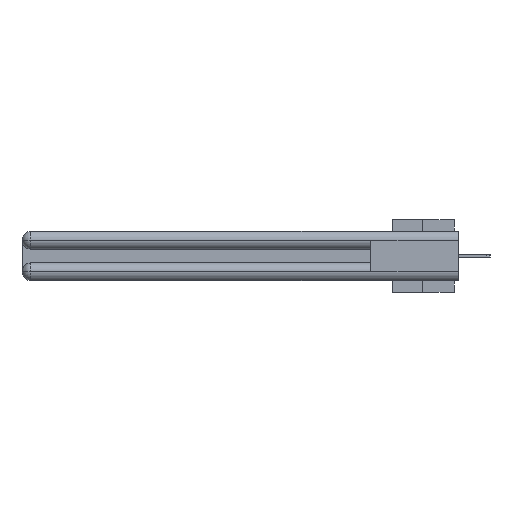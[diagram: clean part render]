
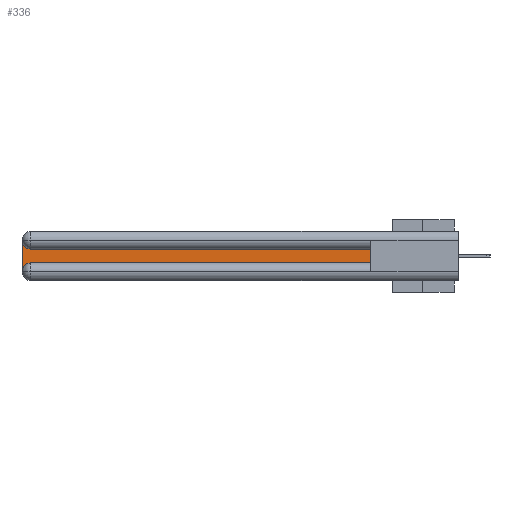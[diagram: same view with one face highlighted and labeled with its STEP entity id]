
A CAD part, left-side view. The second image highlights one B-rep face of the part: STEP entity #336.
In plain terms, the highlighted planar face has unit normal (-1, 0, 0).
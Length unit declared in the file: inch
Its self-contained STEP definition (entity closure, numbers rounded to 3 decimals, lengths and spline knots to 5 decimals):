
#25 = CARTESIAN_POINT ( 'NONE',  ( 0.075, 0.6, -0.1225 ) ) ;
#336 = ADVANCED_FACE ( 'NONE', ( #11092 ), #5457, .F. ) ;
#1108 = DIRECTION ( 'NONE',  ( 1., 0., 0. ) ) ;
#1518 = CARTESIAN_POINT ( 'NONE',  ( 0.075, 3., -0.2175 ) ) ;
#2040 = VERTEX_POINT ( 'NONE', #36958 ) ;
#2284 = DIRECTION ( 'NONE',  ( 1., 0., 0. ) ) ;
#3567 = AXIS2_PLACEMENT_3D ( 'NONE', #16871, #2284, #28264 ) ;
#3638 = VERTEX_POINT ( 'NONE', #27230 ) ;
#3809 = EDGE_CURVE ( 'NONE', #14253, #11996, #15241, .T. ) ;
#4348 = VECTOR ( 'NONE', #9037, 39.37008 ) ;
#4465 = AXIS2_PLACEMENT_3D ( 'NONE', #14529, #25917, #8928 ) ;
#4988 = LINE ( 'NONE', #19565, #5238 ) ;
#5238 = VECTOR ( 'NONE', #22182, 39.37008 ) ;
#5457 = PLANE ( 'NONE',  #3567 ) ;
#5647 = LINE ( 'NONE', #25, #4348 ) ;
#6392 = VECTOR ( 'NONE', #19463, 39.37008 ) ;
#6591 = EDGE_LOOP ( 'NONE', ( #22921, #15003, #34707, #36539, #18831, #24541 ) ) ;
#8928 = DIRECTION ( 'NONE',  ( 0., 0., -1. ) ) ;
#9037 = DIRECTION ( 'NONE',  ( 0., 1., 0. ) ) ;
#9406 = AXIS2_PLACEMENT_3D ( 'NONE', #12530, #1108, #18312 ) ;
#9420 = LINE ( 'NONE', #1518, #22426 ) ;
#10145 = DIRECTION ( 'NONE',  ( 0., 0., -1. ) ) ;
#11092 = FACE_OUTER_BOUND ( 'NONE', #6591, .T. ) ;
#11996 = VERTEX_POINT ( 'NONE', #25471 ) ;
#12530 = CARTESIAN_POINT ( 'NONE',  ( 0.075, 2.94, -0.2775 ) ) ;
#13354 = EDGE_CURVE ( 'NONE', #3638, #21829, #29062, .T. ) ;
#14253 = VERTEX_POINT ( 'NONE', #21542 ) ;
#14529 = CARTESIAN_POINT ( 'NONE',  ( 0.075, 2.94, -0.0625 ) ) ;
#15003 = ORIENTED_EDGE ( 'NONE', *, *, #3809, .T. ) ;
#15241 = CIRCLE ( 'NONE', #4465, 0.06 ) ;
#16393 = EDGE_CURVE ( 'NONE', #34853, #2040, #4988, .T. ) ;
#16871 = CARTESIAN_POINT ( 'NONE',  ( 0.075, 3., -0.1225 ) ) ;
#18312 = DIRECTION ( 'NONE',  ( 0., 0., -1. ) ) ;
#18831 = ORIENTED_EDGE ( 'NONE', *, *, #23660, .T. ) ;
#18912 = CARTESIAN_POINT ( 'NONE',  ( 0.075, 0.6, -0.2175 ) ) ;
#19463 = DIRECTION ( 'NONE',  ( 0., -1., 0. ) ) ;
#19565 = CARTESIAN_POINT ( 'NONE',  ( 0.075, 0.6, -0.2175 ) ) ;
#19652 = LINE ( 'NONE', #18912, #6392 ) ;
#21542 = CARTESIAN_POINT ( 'NONE',  ( 0.075, 2.94, -0.1225 ) ) ;
#21829 = VERTEX_POINT ( 'NONE', #29422 ) ;
#22182 = DIRECTION ( 'NONE',  ( 0., 0., 1. ) ) ;
#22324 = EDGE_CURVE ( 'NONE', #11996, #3638, #9420, .T. ) ;
#22426 = VECTOR ( 'NONE', #10145, 39.37008 ) ;
#22921 = ORIENTED_EDGE ( 'NONE', *, *, #32954, .T. ) ;
#23660 = EDGE_CURVE ( 'NONE', #21829, #34853, #19652, .T. ) ;
#24541 = ORIENTED_EDGE ( 'NONE', *, *, #16393, .T. ) ;
#24563 = CARTESIAN_POINT ( 'NONE',  ( 0.075, 0.6, -0.2175 ) ) ;
#25471 = CARTESIAN_POINT ( 'NONE',  ( 0.075, 3., -0.0625 ) ) ;
#25917 = DIRECTION ( 'NONE',  ( 1., 0., 0. ) ) ;
#27230 = CARTESIAN_POINT ( 'NONE',  ( 0.075, 3., -0.2775 ) ) ;
#28264 = DIRECTION ( 'NONE',  ( 0., 0., -1. ) ) ;
#29062 = CIRCLE ( 'NONE', #9406, 0.06 ) ;
#29422 = CARTESIAN_POINT ( 'NONE',  ( 0.075, 2.94, -0.2175 ) ) ;
#32954 = EDGE_CURVE ( 'NONE', #2040, #14253, #5647, .T. ) ;
#34707 = ORIENTED_EDGE ( 'NONE', *, *, #22324, .T. ) ;
#34853 = VERTEX_POINT ( 'NONE', #24563 ) ;
#36539 = ORIENTED_EDGE ( 'NONE', *, *, #13354, .T. ) ;
#36958 = CARTESIAN_POINT ( 'NONE',  ( 0.075, 0.6, -0.1225 ) ) ;
